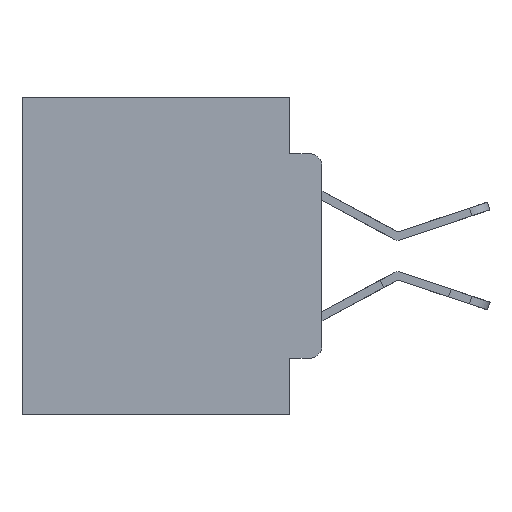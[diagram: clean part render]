
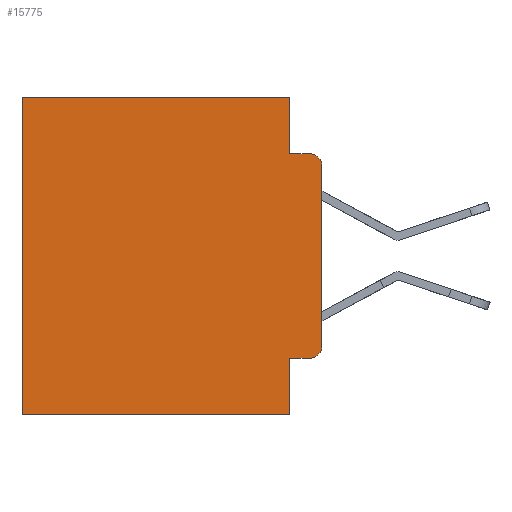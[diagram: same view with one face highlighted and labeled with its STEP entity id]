
A CAD part, left-side view. The second image highlights one B-rep face of the part: STEP entity #15775.
In plain terms, the highlighted planar face has unit normal (-1, 0, 0).
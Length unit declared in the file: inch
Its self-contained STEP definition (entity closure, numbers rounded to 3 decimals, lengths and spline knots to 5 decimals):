
#114 = CARTESIAN_POINT ( 'NONE',  ( 0.298, 0.473, 0. ) ) ;
#280 = LINE ( 'NONE', #18713, #7990 ) ;
#303 = CARTESIAN_POINT ( 'NONE',  ( 0.298, 0.02, -0.0885 ) ) ;
#456 = DIRECTION ( 'NONE',  ( 0., 0., -1. ) ) ;
#470 = EDGE_CURVE ( 'NONE', #1675, #17060, #1039, .T. ) ;
#930 = DIRECTION ( 'NONE',  ( 0., 0., -1. ) ) ;
#955 = AXIS2_PLACEMENT_3D ( 'NONE', #17003, #9758, #930 ) ;
#1039 = LINE ( 'NONE', #7811, #16378 ) ;
#1245 = CARTESIAN_POINT ( 'NONE',  ( 0.298, 0.051, -0.4115 ) ) ;
#1499 = VERTEX_POINT ( 'NONE', #22184 ) ;
#1675 = VERTEX_POINT ( 'NONE', #2793 ) ;
#1707 = VECTOR ( 'NONE', #456, 39.37008 ) ;
#1942 = ORIENTED_EDGE ( 'NONE', *, *, #10167, .T. ) ;
#1978 = LINE ( 'NONE', #13472, #14870 ) ;
#1988 = EDGE_CURVE ( 'NONE', #12120, #16336, #280, .T. ) ;
#2122 = DIRECTION ( 'NONE',  ( 0., -1., 0. ) ) ;
#2793 = CARTESIAN_POINT ( 'NONE',  ( 0.298, 0.051, -0.5 ) ) ;
#3423 = ORIENTED_EDGE ( 'NONE', *, *, #1988, .F. ) ;
#3766 = CARTESIAN_POINT ( 'NONE',  ( 0.298, 0.02, -0.3915 ) ) ;
#3870 = CARTESIAN_POINT ( 'NONE',  ( 0.298, 0.051, -0.0885 ) ) ;
#4090 = VERTEX_POINT ( 'NONE', #303 ) ;
#4763 = CARTESIAN_POINT ( 'NONE',  ( 0.298, 0.02, -0.1085 ) ) ;
#5505 = CARTESIAN_POINT ( 'NONE',  ( 0.298, 0.473, -0.5 ) ) ;
#6420 = DIRECTION ( 'NONE',  ( 0., 0., -1. ) ) ;
#6622 = CARTESIAN_POINT ( 'NONE',  ( 0.298, 0., -0.1085 ) ) ;
#6850 = CIRCLE ( 'NONE', #21989, 0.02 ) ;
#7010 = EDGE_CURVE ( 'NONE', #26142, #4090, #6850, .T. ) ;
#7091 = EDGE_CURVE ( 'NONE', #16336, #4090, #25887, .T. ) ;
#7249 = EDGE_CURVE ( 'NONE', #12120, #1499, #17008, .T. ) ;
#7441 = EDGE_CURVE ( 'NONE', #23717, #1675, #29014, .T. ) ;
#7811 = CARTESIAN_POINT ( 'NONE',  ( 0.298, 0., -0.5 ) ) ;
#7990 = VECTOR ( 'NONE', #25079, 39.37008 ) ;
#8875 = CARTESIAN_POINT ( 'NONE',  ( 0.298, 0.051, 0. ) ) ;
#9283 = ORIENTED_EDGE ( 'NONE', *, *, #7010, .T. ) ;
#9758 = DIRECTION ( 'NONE',  ( 1., 0., 0. ) ) ;
#9907 = FACE_OUTER_BOUND ( 'NONE', #15935, .T. ) ;
#10021 = DIRECTION ( 'NONE',  ( 0., 1., 0. ) ) ;
#10167 = EDGE_CURVE ( 'NONE', #20626, #16115, #27281, .T. ) ;
#10876 = ORIENTED_EDGE ( 'NONE', *, *, #22974, .T. ) ;
#11002 = CARTESIAN_POINT ( 'NONE',  ( 0.298, 0., 0. ) ) ;
#11050 = VECTOR ( 'NONE', #26853, 39.37008 ) ;
#11142 = DIRECTION ( 'NONE',  ( 0., 0., -1. ) ) ;
#11857 = ORIENTED_EDGE ( 'NONE', *, *, #7441, .F. ) ;
#12120 = VERTEX_POINT ( 'NONE', #16502 ) ;
#12270 = ORIENTED_EDGE ( 'NONE', *, *, #470, .F. ) ;
#12345 = CARTESIAN_POINT ( 'NONE',  ( 0.298, 0., -0.3915 ) ) ;
#12713 = DIRECTION ( 'NONE',  ( 0., 1., 0. ) ) ;
#12762 = DIRECTION ( 'NONE',  ( -1., 0., 0. ) ) ;
#13123 = AXIS2_PLACEMENT_3D ( 'NONE', #3766, #12762, #6420 ) ;
#13472 = CARTESIAN_POINT ( 'NONE',  ( 0.298, 0.051, -0.4115 ) ) ;
#13650 = CARTESIAN_POINT ( 'NONE',  ( 0.298, 0.051, -0.0885 ) ) ;
#14870 = VECTOR ( 'NONE', #2122, 39.37008 ) ;
#14897 = VECTOR ( 'NONE', #12713, 39.37008 ) ;
#15775 = ADVANCED_FACE ( 'NONE', ( #9907 ), #16561, .F. ) ;
#15935 = EDGE_LOOP ( 'NONE', ( #25046, #9283, #18239, #3423, #28415, #10876, #12270, #11857, #22007, #1942 ) ) ;
#16115 = VERTEX_POINT ( 'NONE', #12345 ) ;
#16336 = VERTEX_POINT ( 'NONE', #13650 ) ;
#16378 = VECTOR ( 'NONE', #10021, 39.37008 ) ;
#16502 = CARTESIAN_POINT ( 'NONE',  ( 0.298, 0.051, 0. ) ) ;
#16561 = PLANE ( 'NONE',  #955 ) ;
#16564 = DIRECTION ( 'NONE',  ( 0., 0., -1. ) ) ;
#16762 = VECTOR ( 'NONE', #26187, 39.37008 ) ;
#17003 = CARTESIAN_POINT ( 'NONE',  ( 0.298, 0., 0. ) ) ;
#17008 = LINE ( 'NONE', #17159, #14897 ) ;
#17060 = VERTEX_POINT ( 'NONE', #5505 ) ;
#17159 = CARTESIAN_POINT ( 'NONE',  ( 0.298, 0., 0. ) ) ;
#17692 = LINE ( 'NONE', #114, #11050 ) ;
#18239 = ORIENTED_EDGE ( 'NONE', *, *, #7091, .F. ) ;
#18713 = CARTESIAN_POINT ( 'NONE',  ( 0.298, 0.051, 0. ) ) ;
#20626 = VERTEX_POINT ( 'NONE', #28023 ) ;
#20865 = DIRECTION ( 'NONE',  ( -1., 0., 0. ) ) ;
#21989 = AXIS2_PLACEMENT_3D ( 'NONE', #4763, #20865, #16564 ) ;
#22007 = ORIENTED_EDGE ( 'NONE', *, *, #24114, .T. ) ;
#22184 = CARTESIAN_POINT ( 'NONE',  ( 0.298, 0.473, 0. ) ) ;
#22240 = LINE ( 'NONE', #11002, #26191 ) ;
#22974 = EDGE_CURVE ( 'NONE', #1499, #17060, #17692, .T. ) ;
#23394 = EDGE_CURVE ( 'NONE', #26142, #16115, #22240, .T. ) ;
#23717 = VERTEX_POINT ( 'NONE', #1245 ) ;
#24114 = EDGE_CURVE ( 'NONE', #23717, #20626, #1978, .T. ) ;
#25046 = ORIENTED_EDGE ( 'NONE', *, *, #23394, .F. ) ;
#25079 = DIRECTION ( 'NONE',  ( 0., 0., -1. ) ) ;
#25887 = LINE ( 'NONE', #3870, #16762 ) ;
#26142 = VERTEX_POINT ( 'NONE', #6622 ) ;
#26187 = DIRECTION ( 'NONE',  ( 0., -1., 0. ) ) ;
#26191 = VECTOR ( 'NONE', #11142, 39.37008 ) ;
#26853 = DIRECTION ( 'NONE',  ( 0., 0., -1. ) ) ;
#27281 = CIRCLE ( 'NONE', #13123, 0.02 ) ;
#28023 = CARTESIAN_POINT ( 'NONE',  ( 0.298, 0.02, -0.4115 ) ) ;
#28415 = ORIENTED_EDGE ( 'NONE', *, *, #7249, .T. ) ;
#29014 = LINE ( 'NONE', #8875, #1707 ) ;
